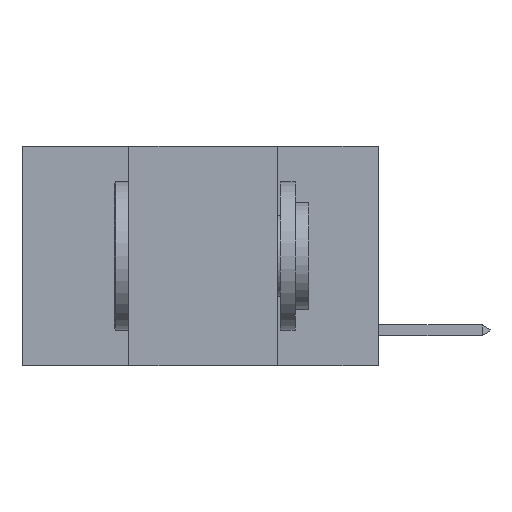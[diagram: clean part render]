
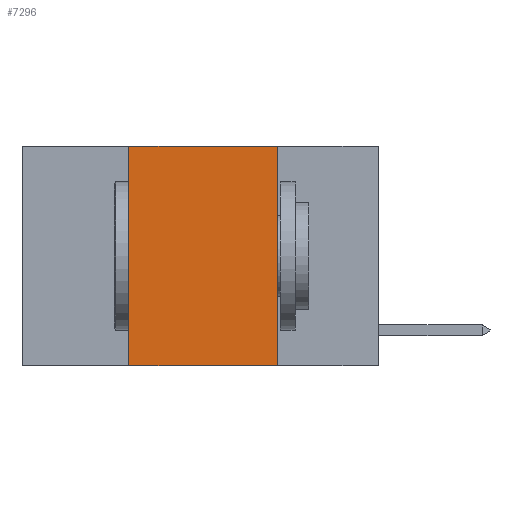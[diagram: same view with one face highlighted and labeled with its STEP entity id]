
A CAD part, left-side view. The second image highlights one B-rep face of the part: STEP entity #7296.
In plain terms, the highlighted planar face has unit normal (-1, 0, 0).
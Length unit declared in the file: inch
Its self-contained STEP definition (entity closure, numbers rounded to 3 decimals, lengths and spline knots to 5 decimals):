
#683 = DIRECTION ( 'NONE',  ( 0., 0., 1. ) ) ;
#1050 = LINE ( 'NONE', #4770, #6928 ) ;
#1475 = ORIENTED_EDGE ( 'NONE', *, *, #4282, .T. ) ;
#1576 = EDGE_LOOP ( 'NONE', ( #12910, #3840, #6590, #1475 ) ) ;
#1967 = DIRECTION ( 'NONE',  ( 0., -1., 0. ) ) ;
#2691 = EDGE_CURVE ( 'NONE', #13942, #11770, #3140, .T. ) ;
#3140 = LINE ( 'NONE', #14364, #8936 ) ;
#3291 = AXIS2_PLACEMENT_3D ( 'NONE', #10706, #3825, #11804 ) ;
#3345 = LINE ( 'NONE', #8909, #6064 ) ;
#3529 = LINE ( 'NONE', #7509, #9326 ) ;
#3825 = DIRECTION ( 'NONE',  ( 1., 0., 0. ) ) ;
#3840 = ORIENTED_EDGE ( 'NONE', *, *, #9236, .F. ) ;
#4282 = EDGE_CURVE ( 'NONE', #13942, #13760, #1050, .T. ) ;
#4770 = CARTESIAN_POINT ( 'NONE',  ( 0., 0.6, -0.37 ) ) ;
#6064 = VECTOR ( 'NONE', #1967, 39.37008 ) ;
#6105 = VERTEX_POINT ( 'NONE', #7250 ) ;
#6109 = PLANE ( 'NONE',  #3291 ) ;
#6590 = ORIENTED_EDGE ( 'NONE', *, *, #2691, .F. ) ;
#6928 = VECTOR ( 'NONE', #12672, 39.37008 ) ;
#7250 = CARTESIAN_POINT ( 'NONE',  ( 0., 0.17, 0. ) ) ;
#7296 = ADVANCED_FACE ( 'NONE', ( #12131 ), #6109, .F. ) ;
#7509 = CARTESIAN_POINT ( 'NONE',  ( 0., 0.17, 0. ) ) ;
#8909 = CARTESIAN_POINT ( 'NONE',  ( 0., 0.6, 0. ) ) ;
#8936 = VECTOR ( 'NONE', #683, 39.37008 ) ;
#8992 = EDGE_CURVE ( 'NONE', #6105, #13760, #3529, .T. ) ;
#9236 = EDGE_CURVE ( 'NONE', #11770, #6105, #3345, .T. ) ;
#9326 = VECTOR ( 'NONE', #13028, 39.37008 ) ;
#9869 = CARTESIAN_POINT ( 'NONE',  ( 0., 0.42, -0.37 ) ) ;
#10706 = CARTESIAN_POINT ( 'NONE',  ( 0., 0.6, 0. ) ) ;
#10810 = CARTESIAN_POINT ( 'NONE',  ( 0., 0.17, -0.37 ) ) ;
#11770 = VERTEX_POINT ( 'NONE', #12289 ) ;
#11804 = DIRECTION ( 'NONE',  ( 0., 0., -1. ) ) ;
#12131 = FACE_OUTER_BOUND ( 'NONE', #1576, .T. ) ;
#12289 = CARTESIAN_POINT ( 'NONE',  ( 0., 0.42, 0. ) ) ;
#12672 = DIRECTION ( 'NONE',  ( 0., -1., 0. ) ) ;
#12910 = ORIENTED_EDGE ( 'NONE', *, *, #8992, .F. ) ;
#13028 = DIRECTION ( 'NONE',  ( 0., 0., -1. ) ) ;
#13760 = VERTEX_POINT ( 'NONE', #10810 ) ;
#13942 = VERTEX_POINT ( 'NONE', #9869 ) ;
#14364 = CARTESIAN_POINT ( 'NONE',  ( 0., 0.42, 0. ) ) ;
